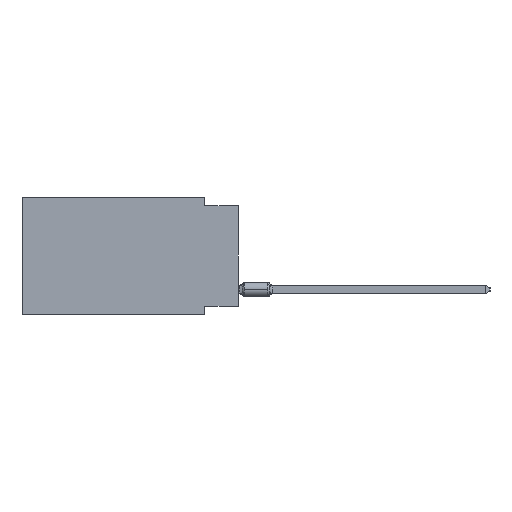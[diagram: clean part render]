
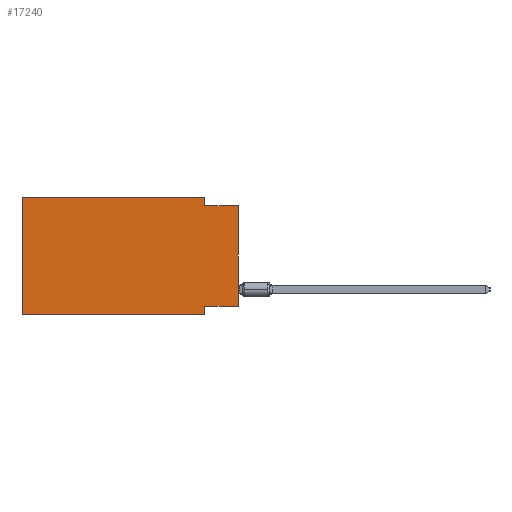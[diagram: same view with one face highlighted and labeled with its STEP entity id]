
A CAD part, left-side view. The second image highlights one B-rep face of the part: STEP entity #17240.
In plain terms, the highlighted planar face has unit normal (-1, 0, 0).
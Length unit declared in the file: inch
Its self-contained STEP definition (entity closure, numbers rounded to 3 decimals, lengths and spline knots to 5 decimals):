
#916 = DIRECTION ( 'NONE',  ( 1., 0., 0. ) ) ;
#1028 = VECTOR ( 'NONE', #19388, 39.37008 ) ;
#1186 = CARTESIAN_POINT ( 'NONE',  ( 0., 0.1, 0. ) ) ;
#1398 = CARTESIAN_POINT ( 'NONE',  ( 0., 0.645, -0.35 ) ) ;
#2622 = EDGE_CURVE ( 'NONE', #13400, #11646, #15511, .T. ) ;
#3273 = CARTESIAN_POINT ( 'NONE',  ( 0., 0.1, -0.35 ) ) ;
#3385 = CARTESIAN_POINT ( 'NONE',  ( 0., 0.645, 0. ) ) ;
#5362 = AXIS2_PLACEMENT_3D ( 'NONE', #44666, #916, #8868 ) ;
#5607 = EDGE_CURVE ( 'NONE', #34519, #11646, #14534, .T. ) ;
#6201 = VECTOR ( 'NONE', #27835, 39.37008 ) ;
#6390 = VERTEX_POINT ( 'NONE', #33594 ) ;
#8616 = FACE_OUTER_BOUND ( 'NONE', #47941, .T. ) ;
#8868 = DIRECTION ( 'NONE',  ( 0., 0., -1. ) ) ;
#9951 = DIRECTION ( 'NONE',  ( 0., 1., 0. ) ) ;
#10463 = DIRECTION ( 'NONE',  ( 0., -1., 0. ) ) ;
#10825 = ORIENTED_EDGE ( 'NONE', *, *, #2622, .F. ) ;
#11513 = ORIENTED_EDGE ( 'NONE', *, *, #36945, .F. ) ;
#11646 = VERTEX_POINT ( 'NONE', #34269 ) ;
#11974 = ORIENTED_EDGE ( 'NONE', *, *, #43764, .F. ) ;
#12061 = VERTEX_POINT ( 'NONE', #25768 ) ;
#13096 = EDGE_CURVE ( 'NONE', #46632, #34462, #15313, .T. ) ;
#13400 = VERTEX_POINT ( 'NONE', #18608 ) ;
#14534 = LINE ( 'NONE', #33722, #24105 ) ;
#15259 = LINE ( 'NONE', #34983, #39993 ) ;
#15313 = LINE ( 'NONE', #32458, #6201 ) ;
#15511 = LINE ( 'NONE', #3273, #1028 ) ;
#15698 = ORIENTED_EDGE ( 'NONE', *, *, #34993, .F. ) ;
#17019 = CARTESIAN_POINT ( 'NONE',  ( 0., 0.1, 0. ) ) ;
#17240 = ADVANCED_FACE ( 'NONE', ( #8616 ), #24436, .F. ) ;
#18608 = CARTESIAN_POINT ( 'NONE',  ( 0., 0.1, -0.325 ) ) ;
#19388 = DIRECTION ( 'NONE',  ( 0., 0., -1. ) ) ;
#19671 = VECTOR ( 'NONE', #46381, 39.37008 ) ;
#21300 = ORIENTED_EDGE ( 'NONE', *, *, #13096, .F. ) ;
#21692 = VECTOR ( 'NONE', #35741, 39.37008 ) ;
#22301 = LINE ( 'NONE', #33358, #36751 ) ;
#24105 = VECTOR ( 'NONE', #10463, 39.37008 ) ;
#24436 = PLANE ( 'NONE',  #5362 ) ;
#24670 = LINE ( 'NONE', #17019, #21692 ) ;
#25206 = ORIENTED_EDGE ( 'NONE', *, *, #45524, .F. ) ;
#25382 = CARTESIAN_POINT ( 'NONE',  ( 0., 0.1, -0.025 ) ) ;
#25768 = CARTESIAN_POINT ( 'NONE',  ( 0., 0., -0.325 ) ) ;
#27835 = DIRECTION ( 'NONE',  ( 0., -1., 0. ) ) ;
#29257 = DIRECTION ( 'NONE',  ( 0., 0., 1. ) ) ;
#29392 = LINE ( 'NONE', #45001, #50195 ) ;
#32458 = CARTESIAN_POINT ( 'NONE',  ( 0., 0., -0.025 ) ) ;
#33358 = CARTESIAN_POINT ( 'NONE',  ( 0., 0., 0. ) ) ;
#33594 = CARTESIAN_POINT ( 'NONE',  ( 0., 0.645, 0. ) ) ;
#33722 = CARTESIAN_POINT ( 'NONE',  ( 0., 0.645, -0.35 ) ) ;
#34269 = CARTESIAN_POINT ( 'NONE',  ( 0., 0.1, -0.35 ) ) ;
#34462 = VERTEX_POINT ( 'NONE', #48710 ) ;
#34519 = VERTEX_POINT ( 'NONE', #1398 ) ;
#34983 = CARTESIAN_POINT ( 'NONE',  ( 0., 0.645, 0. ) ) ;
#34993 = EDGE_CURVE ( 'NONE', #34519, #6390, #15259, .T. ) ;
#35115 = VERTEX_POINT ( 'NONE', #1186 ) ;
#35703 = EDGE_CURVE ( 'NONE', #12061, #34462, #22301, .T. ) ;
#35741 = DIRECTION ( 'NONE',  ( 0., 0., -1. ) ) ;
#36751 = VECTOR ( 'NONE', #29257, 39.37008 ) ;
#36945 = EDGE_CURVE ( 'NONE', #6390, #35115, #46610, .T. ) ;
#39993 = VECTOR ( 'NONE', #43155, 39.37008 ) ;
#43155 = DIRECTION ( 'NONE',  ( 0., 0., 1. ) ) ;
#43764 = EDGE_CURVE ( 'NONE', #12061, #13400, #29392, .T. ) ;
#44666 = CARTESIAN_POINT ( 'NONE',  ( 0., 0.645, 0. ) ) ;
#45001 = CARTESIAN_POINT ( 'NONE',  ( 0., 0., -0.325 ) ) ;
#45495 = ORIENTED_EDGE ( 'NONE', *, *, #35703, .T. ) ;
#45524 = EDGE_CURVE ( 'NONE', #35115, #46632, #24670, .T. ) ;
#46381 = DIRECTION ( 'NONE',  ( 0., -1., 0. ) ) ;
#46610 = LINE ( 'NONE', #3385, #19671 ) ;
#46632 = VERTEX_POINT ( 'NONE', #25382 ) ;
#47369 = ORIENTED_EDGE ( 'NONE', *, *, #5607, .T. ) ;
#47941 = EDGE_LOOP ( 'NONE', ( #45495, #21300, #25206, #11513, #15698, #47369, #10825, #11974 ) ) ;
#48710 = CARTESIAN_POINT ( 'NONE',  ( 0., 0., -0.025 ) ) ;
#50195 = VECTOR ( 'NONE', #9951, 39.37008 ) ;
